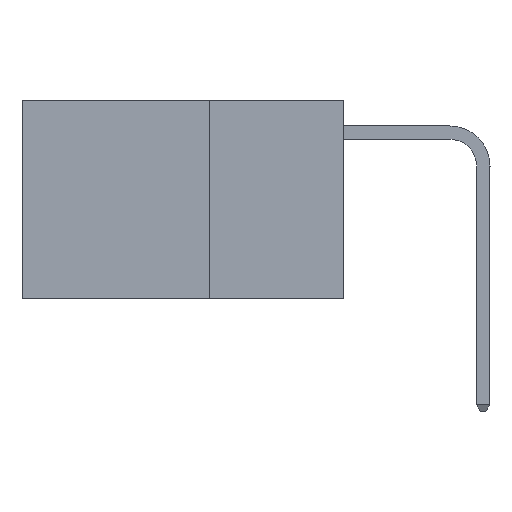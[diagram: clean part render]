
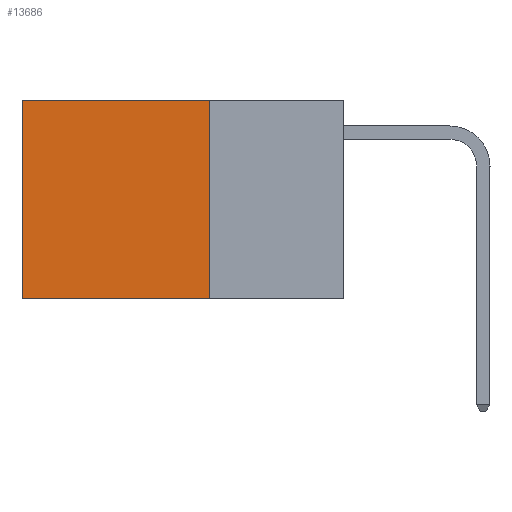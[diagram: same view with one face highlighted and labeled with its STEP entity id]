
A CAD part, left-side view. The second image highlights one B-rep face of the part: STEP entity #13686.
In plain terms, the highlighted planar face has unit normal (-1, 0, 0).
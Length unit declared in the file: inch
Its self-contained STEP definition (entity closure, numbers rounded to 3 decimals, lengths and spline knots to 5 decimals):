
#736 = DIRECTION ( 'NONE',  ( 0., 0., -1. ) ) ;
#855 = FACE_OUTER_BOUND ( 'NONE', #12841, .T. ) ;
#1304 = EDGE_CURVE ( 'NONE', #8738, #7025, #21269, .T. ) ;
#1383 = LINE ( 'NONE', #3953, #11151 ) ;
#2427 = ORIENTED_EDGE ( 'NONE', *, *, #1304, .T. ) ;
#3953 = CARTESIAN_POINT ( 'NONE',  ( 0.2625, 0.25, -0.37 ) ) ;
#4502 = VERTEX_POINT ( 'NONE', #19722 ) ;
#5293 = LINE ( 'NONE', #11217, #19344 ) ;
#6158 = CARTESIAN_POINT ( 'NONE',  ( 0.2625, 0.25, 0. ) ) ;
#6428 = EDGE_CURVE ( 'NONE', #4502, #16047, #12224, .T. ) ;
#7025 = VERTEX_POINT ( 'NONE', #17465 ) ;
#8107 = CARTESIAN_POINT ( 'NONE',  ( 0.2625, 0.25, 0. ) ) ;
#8738 = VERTEX_POINT ( 'NONE', #13127 ) ;
#9956 = DIRECTION ( 'NONE',  ( 0., 0., -1. ) ) ;
#11037 = CARTESIAN_POINT ( 'NONE',  ( 0.2625, 0.6, 0. ) ) ;
#11151 = VECTOR ( 'NONE', #16794, 39.37008 ) ;
#11217 = CARTESIAN_POINT ( 'NONE',  ( 0.2625, 0.25, 0. ) ) ;
#11404 = ORIENTED_EDGE ( 'NONE', *, *, #6428, .F. ) ;
#12090 = AXIS2_PLACEMENT_3D ( 'NONE', #8107, #20923, #9956 ) ;
#12224 = LINE ( 'NONE', #6158, #20252 ) ;
#12841 = EDGE_LOOP ( 'NONE', ( #2427, #20037, #11404, #23571 ) ) ;
#13047 = DIRECTION ( 'NONE',  ( 0., 1., 0. ) ) ;
#13127 = CARTESIAN_POINT ( 'NONE',  ( 0.2625, 0.6, 0. ) ) ;
#13195 = DIRECTION ( 'NONE',  ( 0., 0., -1. ) ) ;
#13686 = ADVANCED_FACE ( 'NONE', ( #855 ), #15417, .F. ) ;
#15417 = PLANE ( 'NONE',  #12090 ) ;
#16047 = VERTEX_POINT ( 'NONE', #19123 ) ;
#16365 = EDGE_CURVE ( 'NONE', #4502, #8738, #5293, .T. ) ;
#16794 = DIRECTION ( 'NONE',  ( 0., 1., 0. ) ) ;
#17465 = CARTESIAN_POINT ( 'NONE',  ( 0.2625, 0.6, -0.37 ) ) ;
#19123 = CARTESIAN_POINT ( 'NONE',  ( 0.2625, 0.25, -0.37 ) ) ;
#19344 = VECTOR ( 'NONE', #13047, 39.37008 ) ;
#19722 = CARTESIAN_POINT ( 'NONE',  ( 0.2625, 0.25, 0. ) ) ;
#20037 = ORIENTED_EDGE ( 'NONE', *, *, #21541, .F. ) ;
#20252 = VECTOR ( 'NONE', #736, 39.37008 ) ;
#20668 = VECTOR ( 'NONE', #13195, 39.37008 ) ;
#20923 = DIRECTION ( 'NONE',  ( 1., 0., 0. ) ) ;
#21269 = LINE ( 'NONE', #11037, #20668 ) ;
#21541 = EDGE_CURVE ( 'NONE', #16047, #7025, #1383, .T. ) ;
#23571 = ORIENTED_EDGE ( 'NONE', *, *, #16365, .T. ) ;
